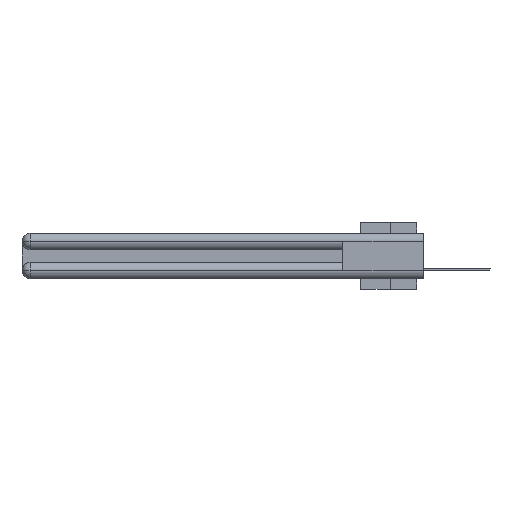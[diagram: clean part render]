
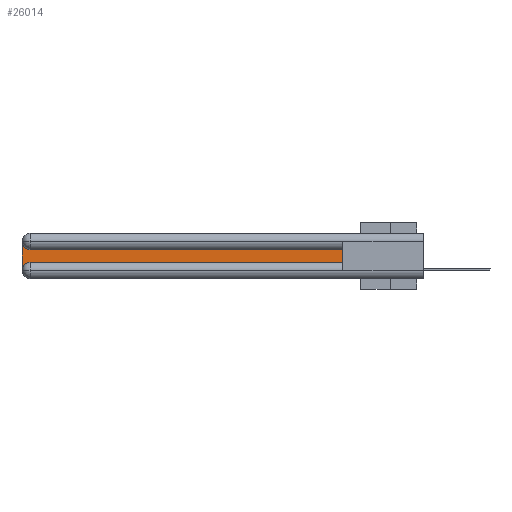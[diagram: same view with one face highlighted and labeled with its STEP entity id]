
A CAD part, left-side view. The second image highlights one B-rep face of the part: STEP entity #26014.
In plain terms, the highlighted planar face has unit normal (-1, 0, 0).
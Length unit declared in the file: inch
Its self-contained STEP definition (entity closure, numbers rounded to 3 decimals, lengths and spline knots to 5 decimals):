
#233 = VERTEX_POINT ( 'NONE', #34270 ) ;
#1238 = DIRECTION ( 'NONE',  ( 0., 1., 0. ) ) ;
#1381 = DIRECTION ( 'NONE',  ( 1., 0., 0. ) ) ;
#2315 = CARTESIAN_POINT ( 'NONE',  ( 0.075, 0.6, -0.2175 ) ) ;
#2750 = DIRECTION ( 'NONE',  ( 0., 0., -1. ) ) ;
#5005 = DIRECTION ( 'NONE',  ( 0., -1., 0. ) ) ;
#5075 = EDGE_CURVE ( 'NONE', #24595, #30344, #19851, .T. ) ;
#5107 = AXIS2_PLACEMENT_3D ( 'NONE', #29660, #1381, #2750 ) ;
#5986 = AXIS2_PLACEMENT_3D ( 'NONE', #10193, #22773, #22379 ) ;
#7209 = EDGE_CURVE ( 'NONE', #28930, #26917, #18132, .T. ) ;
#7525 = VECTOR ( 'NONE', #16337, 39.37008 ) ;
#9543 = EDGE_CURVE ( 'NONE', #26917, #10414, #38623, .T. ) ;
#9647 = EDGE_LOOP ( 'NONE', ( #39439, #20951, #13060, #40450, #10887, #20266 ) ) ;
#10193 = CARTESIAN_POINT ( 'NONE',  ( 0.075, 2.94, -0.0625 ) ) ;
#10414 = VERTEX_POINT ( 'NONE', #27688 ) ;
#10887 = ORIENTED_EDGE ( 'NONE', *, *, #26200, .T. ) ;
#13060 = ORIENTED_EDGE ( 'NONE', *, *, #5075, .T. ) ;
#13071 = FACE_OUTER_BOUND ( 'NONE', #9647, .T. ) ;
#13825 = CARTESIAN_POINT ( 'NONE',  ( 0.075, 0.6, -0.1225 ) ) ;
#16123 = CARTESIAN_POINT ( 'NONE',  ( 0.075, 0.6, -0.2175 ) ) ;
#16236 = AXIS2_PLACEMENT_3D ( 'NONE', #34561, #31667, #40763 ) ;
#16337 = DIRECTION ( 'NONE',  ( 0., 0., -1. ) ) ;
#16631 = EDGE_CURVE ( 'NONE', #10414, #24595, #25760, .T. ) ;
#18132 = LINE ( 'NONE', #18334, #29672 ) ;
#18334 = CARTESIAN_POINT ( 'NONE',  ( 0.075, 0.6, -0.2175 ) ) ;
#19851 = LINE ( 'NONE', #38869, #7525 ) ;
#20241 = CIRCLE ( 'NONE', #5107, 0.06 ) ;
#20266 = ORIENTED_EDGE ( 'NONE', *, *, #7209, .T. ) ;
#20599 = VECTOR ( 'NONE', #1238, 39.37008 ) ;
#20951 = ORIENTED_EDGE ( 'NONE', *, *, #16631, .T. ) ;
#22379 = DIRECTION ( 'NONE',  ( 0., 0., -1. ) ) ;
#22773 = DIRECTION ( 'NONE',  ( 1., 0., 0. ) ) ;
#23225 = CARTESIAN_POINT ( 'NONE',  ( 0.075, 0.6, -0.1225 ) ) ;
#23618 = CARTESIAN_POINT ( 'NONE',  ( 0.075, 3., -0.0625 ) ) ;
#24595 = VERTEX_POINT ( 'NONE', #23618 ) ;
#25664 = PLANE ( 'NONE',  #16236 ) ;
#25760 = CIRCLE ( 'NONE', #5986, 0.06 ) ;
#26014 = ADVANCED_FACE ( 'NONE', ( #13071 ), #25664, .F. ) ;
#26200 = EDGE_CURVE ( 'NONE', #233, #28930, #27294, .T. ) ;
#26917 = VERTEX_POINT ( 'NONE', #23225 ) ;
#27294 = LINE ( 'NONE', #2315, #28101 ) ;
#27688 = CARTESIAN_POINT ( 'NONE',  ( 0.075, 2.94, -0.1225 ) ) ;
#28101 = VECTOR ( 'NONE', #5005, 39.37008 ) ;
#28930 = VERTEX_POINT ( 'NONE', #16123 ) ;
#29660 = CARTESIAN_POINT ( 'NONE',  ( 0.075, 2.94, -0.2775 ) ) ;
#29672 = VECTOR ( 'NONE', #40257, 39.37008 ) ;
#30344 = VERTEX_POINT ( 'NONE', #38846 ) ;
#31667 = DIRECTION ( 'NONE',  ( 1., 0., 0. ) ) ;
#34270 = CARTESIAN_POINT ( 'NONE',  ( 0.075, 2.94, -0.2175 ) ) ;
#34561 = CARTESIAN_POINT ( 'NONE',  ( 0.075, 3., -0.1225 ) ) ;
#37618 = EDGE_CURVE ( 'NONE', #30344, #233, #20241, .T. ) ;
#38623 = LINE ( 'NONE', #13825, #20599 ) ;
#38846 = CARTESIAN_POINT ( 'NONE',  ( 0.075, 3., -0.2775 ) ) ;
#38869 = CARTESIAN_POINT ( 'NONE',  ( 0.075, 3., -0.2175 ) ) ;
#39439 = ORIENTED_EDGE ( 'NONE', *, *, #9543, .T. ) ;
#40257 = DIRECTION ( 'NONE',  ( 0., 0., 1. ) ) ;
#40450 = ORIENTED_EDGE ( 'NONE', *, *, #37618, .T. ) ;
#40763 = DIRECTION ( 'NONE',  ( 0., 0., -1. ) ) ;
